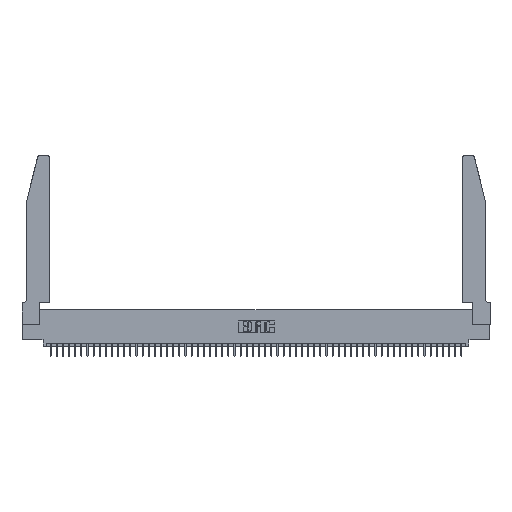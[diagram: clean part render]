
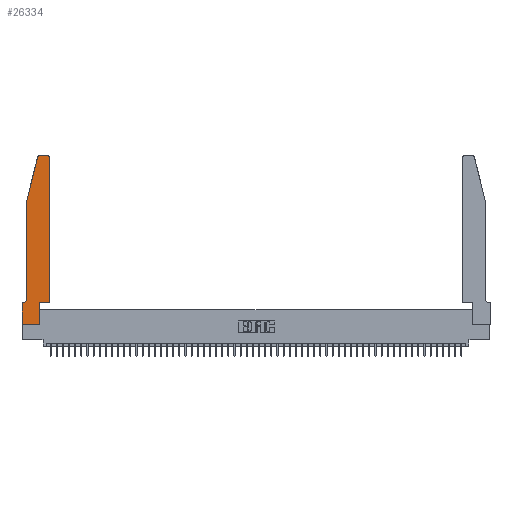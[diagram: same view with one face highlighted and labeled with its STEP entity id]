
A CAD part, top view. The second image highlights one B-rep face of the part: STEP entity #26334.
In plain terms, the highlighted planar face has unit normal (0, 0, 1).
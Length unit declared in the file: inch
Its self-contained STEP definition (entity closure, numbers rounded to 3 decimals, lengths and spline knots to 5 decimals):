
#704 = CARTESIAN_POINT ( 'NONE',  ( 0.4205, 2.72, 0.37 ) ) ;
#2267 = VECTOR ( 'NONE', #14209, 39.37008 ) ;
#2502 = EDGE_CURVE ( 'NONE', #29962, #41288, #48241, .T. ) ;
#3220 = LINE ( 'NONE', #53021, #38374 ) ;
#4161 = VECTOR ( 'NONE', #48020, 39.37008 ) ;
#5060 = DIRECTION ( 'NONE',  ( 1., 0., 0. ) ) ;
#5442 = DIRECTION ( 'NONE',  ( 0., -1., 0. ) ) ;
#6854 = DIRECTION ( 'NONE',  ( 0., 1., 0. ) ) ;
#7624 = ORIENTED_EDGE ( 'NONE', *, *, #2502, .T. ) ;
#7796 = VERTEX_POINT ( 'NONE', #33168 ) ;
#7884 = EDGE_CURVE ( 'NONE', #41024, #9568, #17331, .T. ) ;
#9568 = VERTEX_POINT ( 'NONE', #32586 ) ;
#9893 = CARTESIAN_POINT ( 'NONE',  ( 0.2605, 2.75, 0.37 ) ) ;
#10509 = EDGE_CURVE ( 'NONE', #17473, #17650, #45035, .T. ) ;
#10946 = ORIENTED_EDGE ( 'NONE', *, *, #7884, .T. ) ;
#11041 = VERTEX_POINT ( 'NONE', #12843 ) ;
#11345 = EDGE_CURVE ( 'NONE', #21138, #29962, #17841, .T. ) ;
#12086 = VERTEX_POINT ( 'NONE', #19104 ) ;
#12843 = CARTESIAN_POINT ( 'NONE',  ( 0.4205, 2.75, 0.37 ) ) ;
#12863 = LINE ( 'NONE', #52594, #21501 ) ;
#14018 = ORIENTED_EDGE ( 'NONE', *, *, #49960, .T. ) ;
#14209 = DIRECTION ( 'NONE',  ( -1., 0., 0. ) ) ;
#14374 = ORIENTED_EDGE ( 'NONE', *, *, #26773, .T. ) ;
#16246 = ORIENTED_EDGE ( 'NONE', *, *, #32646, .T. ) ;
#16924 = DIRECTION ( 'NONE',  ( 0., 0., -1. ) ) ;
#17331 = CIRCLE ( 'NONE', #51803, 0.07 ) ;
#17473 = VERTEX_POINT ( 'NONE', #34877 ) ;
#17650 = VERTEX_POINT ( 'NONE', #35983 ) ;
#17841 = CIRCLE ( 'NONE', #48053, 0.03 ) ;
#18214 = DIRECTION ( 'NONE',  ( 0., 1., 0. ) ) ;
#18798 = VERTEX_POINT ( 'NONE', #26781 ) ;
#19104 = CARTESIAN_POINT ( 'NONE',  ( 0.4505, 2.72, 0.37 ) ) ;
#19541 = CARTESIAN_POINT ( 'NONE',  ( 0.4505, 0.35, 0.37 ) ) ;
#19718 = AXIS2_PLACEMENT_3D ( 'NONE', #704, #30454, #5060 ) ;
#20266 = DIRECTION ( 'NONE',  ( 0., 0., 1. ) ) ;
#20661 = DIRECTION ( 'NONE',  ( 1., 0., 0. ) ) ;
#21138 = VERTEX_POINT ( 'NONE', #47091 ) ;
#21501 = VECTOR ( 'NONE', #44168, 39.37008 ) ;
#22778 = ORIENTED_EDGE ( 'NONE', *, *, #52989, .T. ) ;
#23086 = CARTESIAN_POINT ( 'NONE',  ( 0.4505, 0.35, 0.37 ) ) ;
#25059 = ORIENTED_EDGE ( 'NONE', *, *, #47231, .T. ) ;
#25773 = VECTOR ( 'NONE', #37573, 39.37008 ) ;
#25842 = VECTOR ( 'NONE', #52543, 39.37008 ) ;
#26334 = ADVANCED_FACE ( 'NONE', ( #47004 ), #41691, .T. ) ;
#26527 = CARTESIAN_POINT ( 'NONE',  ( 0.2865, 0.35, 0.37 ) ) ;
#26762 = LINE ( 'NONE', #43804, #4161 ) ;
#26773 = EDGE_CURVE ( 'NONE', #17650, #18798, #3220, .T. ) ;
#26781 = CARTESIAN_POINT ( 'NONE',  ( 0.2865, 0., 0.37 ) ) ;
#27808 = DIRECTION ( 'NONE',  ( 1., 0., 0. ) ) ;
#28906 = CARTESIAN_POINT ( 'NONE',  ( 0.4505, 0.35, 0.37 ) ) ;
#29457 = EDGE_CURVE ( 'NONE', #54736, #12086, #42991, .T. ) ;
#29962 = VERTEX_POINT ( 'NONE', #46684 ) ;
#30036 = EDGE_LOOP ( 'NONE', ( #25059, #43380, #7624, #43310, #10946, #50788, #48600, #14374, #16246, #14018, #48844, #22778 ) ) ;
#30454 = DIRECTION ( 'NONE',  ( 0., 0., 1. ) ) ;
#30827 = CARTESIAN_POINT ( 'NONE',  ( 0., 0., 0.37 ) ) ;
#32586 = CARTESIAN_POINT ( 'NONE',  ( 0.0055, 0.35, 0.37 ) ) ;
#32646 = EDGE_CURVE ( 'NONE', #18798, #7796, #51197, .T. ) ;
#32924 = AXIS2_PLACEMENT_3D ( 'NONE', #37434, #45933, #20661 ) ;
#33068 = VECTOR ( 'NONE', #6854, 39.37008 ) ;
#33168 = CARTESIAN_POINT ( 'NONE',  ( 0.2865, 0.35, 0.37 ) ) ;
#33310 = CARTESIAN_POINT ( 'NONE',  ( 0.0755, 2., 0.37 ) ) ;
#34877 = CARTESIAN_POINT ( 'NONE',  ( 0., 0.35, 0.37 ) ) ;
#35894 = EDGE_CURVE ( 'NONE', #9568, #17473, #26762, .T. ) ;
#35983 = CARTESIAN_POINT ( 'NONE',  ( 0., 0., 0.37 ) ) ;
#36149 = LINE ( 'NONE', #9893, #2267 ) ;
#37434 = CARTESIAN_POINT ( 'NONE',  ( 0., 0.35, 0.37 ) ) ;
#37573 = DIRECTION ( 'NONE',  ( -0.239, -0.971, 0. ) ) ;
#38374 = VECTOR ( 'NONE', #27808, 39.37008 ) ;
#41024 = VERTEX_POINT ( 'NONE', #41787 ) ;
#41288 = VERTEX_POINT ( 'NONE', #47826 ) ;
#41691 = PLANE ( 'NONE',  #32924 ) ;
#41787 = CARTESIAN_POINT ( 'NONE',  ( 0.0755, 0.42, 0.37 ) ) ;
#42225 = CARTESIAN_POINT ( 'NONE',  ( 0.0055, 0.42, 0.37 ) ) ;
#42991 = LINE ( 'NONE', #19541, #33068 ) ;
#43310 = ORIENTED_EDGE ( 'NONE', *, *, #46748, .T. ) ;
#43380 = ORIENTED_EDGE ( 'NONE', *, *, #11345, .T. ) ;
#43804 = CARTESIAN_POINT ( 'NONE',  ( 0.0755, 0.35, 0.37 ) ) ;
#44168 = DIRECTION ( 'NONE',  ( 0., -1., 0. ) ) ;
#45035 = LINE ( 'NONE', #30827, #47652 ) ;
#45530 = CARTESIAN_POINT ( 'NONE',  ( 0.284, 2.72, 0.37 ) ) ;
#45933 = DIRECTION ( 'NONE',  ( 0., 0., 1. ) ) ;
#46447 = DIRECTION ( 'NONE',  ( -1., 0., 0. ) ) ;
#46684 = CARTESIAN_POINT ( 'NONE',  ( 0.25487, 2.72718, 0.37 ) ) ;
#46748 = EDGE_CURVE ( 'NONE', #41288, #41024, #12863, .T. ) ;
#47004 = FACE_OUTER_BOUND ( 'NONE', #30036, .T. ) ;
#47091 = CARTESIAN_POINT ( 'NONE',  ( 0.284, 2.75, 0.37 ) ) ;
#47231 = EDGE_CURVE ( 'NONE', #11041, #21138, #36149, .T. ) ;
#47652 = VECTOR ( 'NONE', #5442, 39.37008 ) ;
#47826 = CARTESIAN_POINT ( 'NONE',  ( 0.0755, 2., 0.37 ) ) ;
#48020 = DIRECTION ( 'NONE',  ( -1., 0., 0. ) ) ;
#48053 = AXIS2_PLACEMENT_3D ( 'NONE', #45530, #20266, #49723 ) ;
#48241 = LINE ( 'NONE', #33310, #25773 ) ;
#48307 = LINE ( 'NONE', #23086, #25842 ) ;
#48600 = ORIENTED_EDGE ( 'NONE', *, *, #10509, .T. ) ;
#48844 = ORIENTED_EDGE ( 'NONE', *, *, #29457, .T. ) ;
#49723 = DIRECTION ( 'NONE',  ( 1., 0., 0. ) ) ;
#49901 = VECTOR ( 'NONE', #18214, 39.37008 ) ;
#49960 = EDGE_CURVE ( 'NONE', #7796, #54736, #48307, .T. ) ;
#50741 = CIRCLE ( 'NONE', #19718, 0.03 ) ;
#50788 = ORIENTED_EDGE ( 'NONE', *, *, #35894, .T. ) ;
#51197 = LINE ( 'NONE', #26527, #49901 ) ;
#51803 = AXIS2_PLACEMENT_3D ( 'NONE', #42225, #16924, #46447 ) ;
#52543 = DIRECTION ( 'NONE',  ( 1., 0., 0. ) ) ;
#52594 = CARTESIAN_POINT ( 'NONE',  ( 0.0755, 2., 0.37 ) ) ;
#52989 = EDGE_CURVE ( 'NONE', #12086, #11041, #50741, .T. ) ;
#53021 = CARTESIAN_POINT ( 'NONE',  ( 0., 0., 0.37 ) ) ;
#54736 = VERTEX_POINT ( 'NONE', #28906 ) ;
